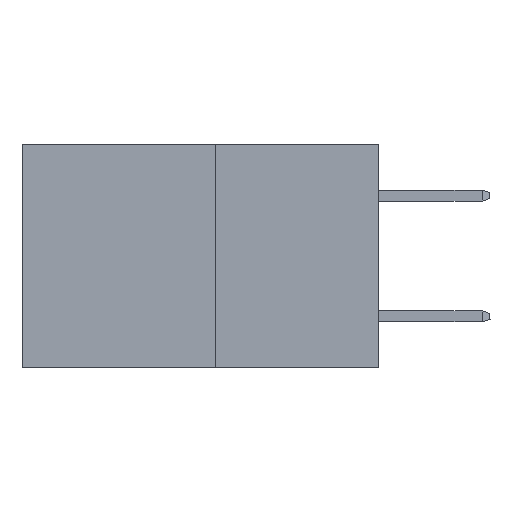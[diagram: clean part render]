
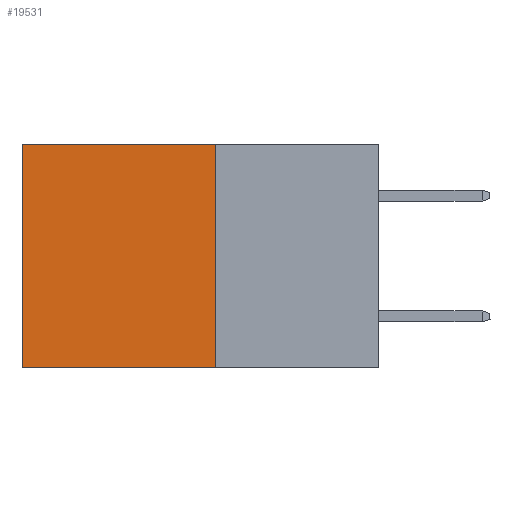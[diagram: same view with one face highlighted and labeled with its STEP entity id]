
A CAD part, left-side view. The second image highlights one B-rep face of the part: STEP entity #19531.
In plain terms, the highlighted planar face has unit normal (-1, 0, 0).
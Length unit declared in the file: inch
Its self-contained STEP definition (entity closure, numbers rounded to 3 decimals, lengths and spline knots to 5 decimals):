
#1409 = DIRECTION ( 'NONE',  ( 0., 1., 0. ) ) ;
#1430 = DIRECTION ( 'NONE',  ( 1., 0., 0. ) ) ;
#1478 = EDGE_CURVE ( 'NONE', #2299, #23764, #16747, .T. ) ;
#2187 = ORIENTED_EDGE ( 'NONE', *, *, #20124, .F. ) ;
#2299 = VERTEX_POINT ( 'NONE', #20598 ) ;
#3591 = DIRECTION ( 'NONE',  ( 0., 1., 0. ) ) ;
#5936 = ORIENTED_EDGE ( 'NONE', *, *, #13000, .F. ) ;
#6401 = LINE ( 'NONE', #25583, #21742 ) ;
#7387 = CARTESIAN_POINT ( 'NONE',  ( 0.277, 0.27, -0.37 ) ) ;
#8547 = VECTOR ( 'NONE', #12293, 39.37008 ) ;
#9771 = CARTESIAN_POINT ( 'NONE',  ( 0.277, 0.27, 0. ) ) ;
#10499 = FACE_OUTER_BOUND ( 'NONE', #10596, .T. ) ;
#10596 = EDGE_LOOP ( 'NONE', ( #12996, #2187, #5936, #23011 ) ) ;
#10627 = CARTESIAN_POINT ( 'NONE',  ( 0.277, 0.27, -0.37 ) ) ;
#12044 = VERTEX_POINT ( 'NONE', #9771 ) ;
#12293 = DIRECTION ( 'NONE',  ( 0., 0., -1. ) ) ;
#12996 = ORIENTED_EDGE ( 'NONE', *, *, #1478, .T. ) ;
#13000 = EDGE_CURVE ( 'NONE', #12044, #24972, #24564, .T. ) ;
#13299 = VECTOR ( 'NONE', #1409, 39.37008 ) ;
#13924 = LINE ( 'NONE', #25406, #13299 ) ;
#14619 = CARTESIAN_POINT ( 'NONE',  ( 0.277, 0.59, -0.37 ) ) ;
#15191 = CARTESIAN_POINT ( 'NONE',  ( 0.277, 0.27, -0.37 ) ) ;
#15264 = EDGE_CURVE ( 'NONE', #12044, #2299, #6401, .T. ) ;
#15330 = PLANE ( 'NONE',  #21694 ) ;
#15409 = DIRECTION ( 'NONE',  ( 0., 0., -1. ) ) ;
#16126 = VECTOR ( 'NONE', #17772, 39.37008 ) ;
#16747 = LINE ( 'NONE', #14619, #16126 ) ;
#17772 = DIRECTION ( 'NONE',  ( 0., 0., -1. ) ) ;
#19531 = ADVANCED_FACE ( 'NONE', ( #10499 ), #15330, .F. ) ;
#20124 = EDGE_CURVE ( 'NONE', #24972, #23764, #13924, .T. ) ;
#20598 = CARTESIAN_POINT ( 'NONE',  ( 0.277, 0.59, 0. ) ) ;
#21694 = AXIS2_PLACEMENT_3D ( 'NONE', #7387, #1430, #15409 ) ;
#21742 = VECTOR ( 'NONE', #3591, 39.37008 ) ;
#23011 = ORIENTED_EDGE ( 'NONE', *, *, #15264, .T. ) ;
#23764 = VERTEX_POINT ( 'NONE', #24120 ) ;
#24120 = CARTESIAN_POINT ( 'NONE',  ( 0.277, 0.59, -0.37 ) ) ;
#24564 = LINE ( 'NONE', #10627, #8547 ) ;
#24972 = VERTEX_POINT ( 'NONE', #15191 ) ;
#25406 = CARTESIAN_POINT ( 'NONE',  ( 0.277, 0.27, -0.37 ) ) ;
#25583 = CARTESIAN_POINT ( 'NONE',  ( 0.277, 0.27, 0. ) ) ;
